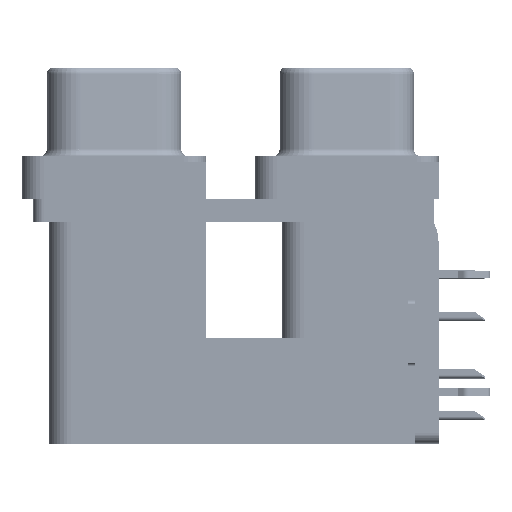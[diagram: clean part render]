
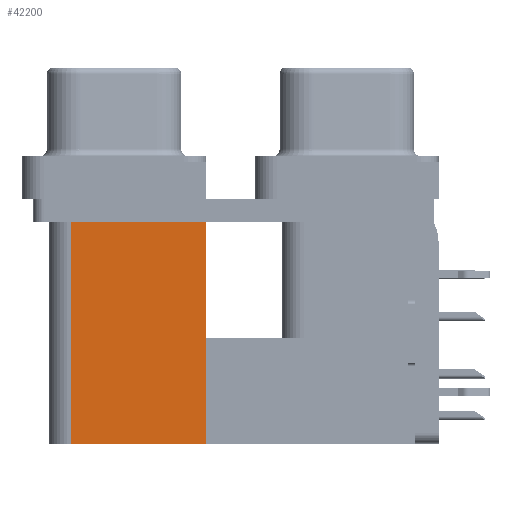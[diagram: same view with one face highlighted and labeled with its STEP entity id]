
A CAD part, left-side view. The second image highlights one B-rep face of the part: STEP entity #42200.
In plain terms, the highlighted planar face has unit normal (-1, 0, 0).
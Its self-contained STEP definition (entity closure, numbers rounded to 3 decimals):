
#1979 = CARTESIAN_POINT ( 'NONE',  ( 3.79, 18.8, -19.2 ) ) ;
#2846 = VECTOR ( 'NONE', #23042, 1000. ) ;
#4762 = PLANE ( 'NONE',  #31279 ) ;
#5302 = VERTEX_POINT ( 'NONE', #25443 ) ;
#5558 = DIRECTION ( 'NONE',  ( 0., 1., 0. ) ) ;
#6599 = CARTESIAN_POINT ( 'NONE',  ( 3.79, 9.6, -19.2 ) ) ;
#7189 = LINE ( 'NONE', #19630, #19716 ) ;
#10147 = ORIENTED_EDGE ( 'NONE', *, *, #49890, .T. ) ;
#10504 = CARTESIAN_POINT ( 'NONE',  ( 3.79, 18.8, -2.5 ) ) ;
#12320 = FACE_OUTER_BOUND ( 'NONE', #18202, .T. ) ;
#12852 = VERTEX_POINT ( 'NONE', #1979 ) ;
#13047 = ORIENTED_EDGE ( 'NONE', *, *, #28759, .F. ) ;
#13648 = CARTESIAN_POINT ( 'NONE',  ( 3.79, 9.6, -19.2 ) ) ;
#18202 = EDGE_LOOP ( 'NONE', ( #42157, #32447, #13047, #10147 ) ) ;
#18709 = LINE ( 'NONE', #35229, #2846 ) ;
#19630 = CARTESIAN_POINT ( 'NONE',  ( 3.79, 9.6, -2.5 ) ) ;
#19716 = VECTOR ( 'NONE', #36149, 1000. ) ;
#23042 = DIRECTION ( 'NONE',  ( 0., 0., 1. ) ) ;
#25443 = CARTESIAN_POINT ( 'NONE',  ( 3.79, 9.6, -2.5 ) ) ;
#28759 = EDGE_CURVE ( 'NONE', #45367, #12852, #41821, .T. ) ;
#28863 = CARTESIAN_POINT ( 'NONE',  ( 3.79, 9.6, -19.2 ) ) ;
#31279 = AXIS2_PLACEMENT_3D ( 'NONE', #28863, #41551, #45889 ) ;
#32301 = CARTESIAN_POINT ( 'NONE',  ( 3.79, 18.8, -19.2 ) ) ;
#32447 = ORIENTED_EDGE ( 'NONE', *, *, #45500, .F. ) ;
#34635 = EDGE_CURVE ( 'NONE', #5302, #37244, #7189, .T. ) ;
#35229 = CARTESIAN_POINT ( 'NONE',  ( 3.79, 9.6, -19.2 ) ) ;
#36149 = DIRECTION ( 'NONE',  ( 0., 1., 0. ) ) ;
#37244 = VERTEX_POINT ( 'NONE', #10504 ) ;
#41551 = DIRECTION ( 'NONE',  ( 1., 0., 0. ) ) ;
#41821 = LINE ( 'NONE', #13648, #45323 ) ;
#42157 = ORIENTED_EDGE ( 'NONE', *, *, #34635, .T. ) ;
#42200 = ADVANCED_FACE ( 'NONE', ( #12320 ), #4762, .F. ) ;
#44544 = VECTOR ( 'NONE', #52613, 1000. ) ;
#45022 = LINE ( 'NONE', #32301, #44544 ) ;
#45323 = VECTOR ( 'NONE', #5558, 1000. ) ;
#45367 = VERTEX_POINT ( 'NONE', #6599 ) ;
#45500 = EDGE_CURVE ( 'NONE', #12852, #37244, #45022, .T. ) ;
#45889 = DIRECTION ( 'NONE',  ( 0., 0., -1. ) ) ;
#49890 = EDGE_CURVE ( 'NONE', #45367, #5302, #18709, .T. ) ;
#52613 = DIRECTION ( 'NONE',  ( 0., 0., 1. ) ) ;
